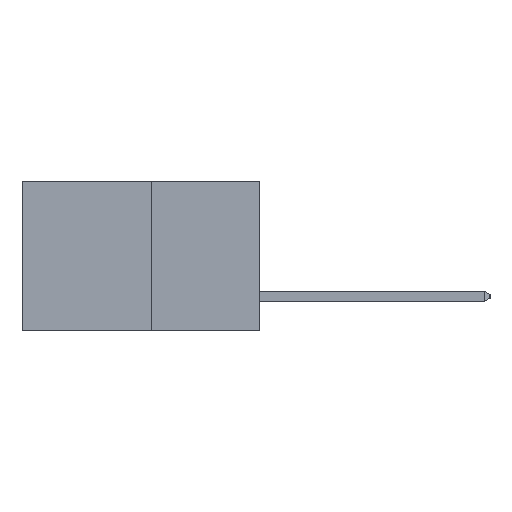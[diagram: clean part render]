
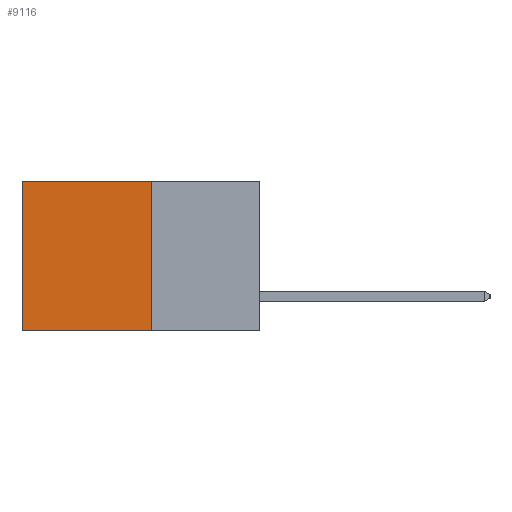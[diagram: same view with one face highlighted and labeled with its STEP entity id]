
A CAD part, left-side view. The second image highlights one B-rep face of the part: STEP entity #9116.
In plain terms, the highlighted planar face has unit normal (-1, 0, 0).
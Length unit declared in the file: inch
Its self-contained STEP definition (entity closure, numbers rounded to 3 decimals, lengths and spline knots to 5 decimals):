
#248 = CARTESIAN_POINT ( 'NONE',  ( 0.277, 0.27, 0. ) ) ;
#459 = LINE ( 'NONE', #1611, #9277 ) ;
#680 = CARTESIAN_POINT ( 'NONE',  ( 0.277, 0.59, -0.37 ) ) ;
#1568 = DIRECTION ( 'NONE',  ( 0., 1., 0. ) ) ;
#1611 = CARTESIAN_POINT ( 'NONE',  ( 0.277, 0.27, 0. ) ) ;
#1745 = EDGE_CURVE ( 'NONE', #10313, #10177, #7828, .T. ) ;
#1840 = EDGE_LOOP ( 'NONE', ( #3363, #5572, #5403, #5447 ) ) ;
#1890 = CARTESIAN_POINT ( 'NONE',  ( 0.277, 0.27, -0.37 ) ) ;
#2498 = VECTOR ( 'NONE', #10423, 39.37008 ) ;
#2738 = PLANE ( 'NONE',  #9276 ) ;
#2799 = VERTEX_POINT ( 'NONE', #5344 ) ;
#3315 = EDGE_CURVE ( 'NONE', #8219, #10313, #459, .T. ) ;
#3363 = ORIENTED_EDGE ( 'NONE', *, *, #1745, .T. ) ;
#3628 = CARTESIAN_POINT ( 'NONE',  ( 0.277, 0.27, -0.37 ) ) ;
#3710 = DIRECTION ( 'NONE',  ( 0., 1., 0. ) ) ;
#3748 = CARTESIAN_POINT ( 'NONE',  ( 0.277, 0.59, -0.37 ) ) ;
#3984 = FACE_OUTER_BOUND ( 'NONE', #1840, .T. ) ;
#4044 = DIRECTION ( 'NONE',  ( 0., 0., -1. ) ) ;
#4803 = CARTESIAN_POINT ( 'NONE',  ( 0.277, 0.27, -0.37 ) ) ;
#5325 = DIRECTION ( 'NONE',  ( 0., 0., -1. ) ) ;
#5344 = CARTESIAN_POINT ( 'NONE',  ( 0.277, 0.27, -0.37 ) ) ;
#5403 = ORIENTED_EDGE ( 'NONE', *, *, #8257, .F. ) ;
#5447 = ORIENTED_EDGE ( 'NONE', *, *, #3315, .T. ) ;
#5572 = ORIENTED_EDGE ( 'NONE', *, *, #9805, .F. ) ;
#6118 = VECTOR ( 'NONE', #3710, 39.37008 ) ;
#7828 = LINE ( 'NONE', #3748, #9881 ) ;
#8029 = LINE ( 'NONE', #1890, #6118 ) ;
#8219 = VERTEX_POINT ( 'NONE', #248 ) ;
#8257 = EDGE_CURVE ( 'NONE', #8219, #2799, #9160, .T. ) ;
#9116 = ADVANCED_FACE ( 'NONE', ( #3984 ), #2738, .F. ) ;
#9160 = LINE ( 'NONE', #4803, #2498 ) ;
#9276 = AXIS2_PLACEMENT_3D ( 'NONE', #3628, #10123, #5325 ) ;
#9277 = VECTOR ( 'NONE', #1568, 39.37008 ) ;
#9354 = CARTESIAN_POINT ( 'NONE',  ( 0.277, 0.59, 0. ) ) ;
#9805 = EDGE_CURVE ( 'NONE', #2799, #10177, #8029, .T. ) ;
#9881 = VECTOR ( 'NONE', #4044, 39.37008 ) ;
#10123 = DIRECTION ( 'NONE',  ( 1., 0., 0. ) ) ;
#10177 = VERTEX_POINT ( 'NONE', #680 ) ;
#10313 = VERTEX_POINT ( 'NONE', #9354 ) ;
#10423 = DIRECTION ( 'NONE',  ( 0., 0., -1. ) ) ;
